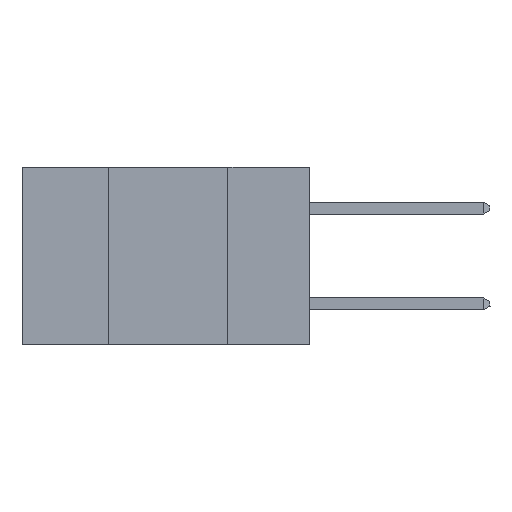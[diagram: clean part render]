
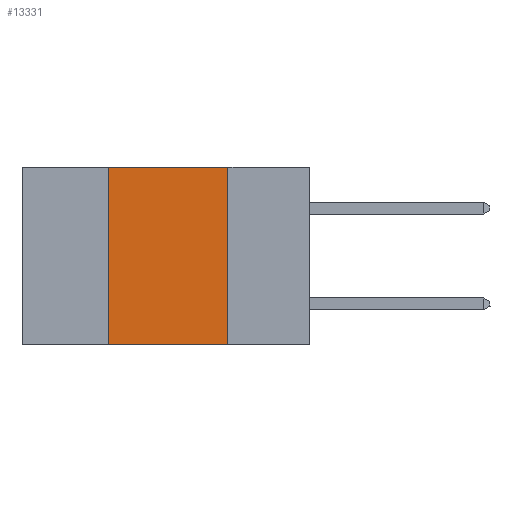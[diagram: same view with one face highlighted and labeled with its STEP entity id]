
A CAD part, left-side view. The second image highlights one B-rep face of the part: STEP entity #13331.
In plain terms, the highlighted planar face has unit normal (-1, 0, 0).
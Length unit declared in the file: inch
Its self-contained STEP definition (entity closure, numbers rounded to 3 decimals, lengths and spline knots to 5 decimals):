
#388 = ORIENTED_EDGE ( 'NONE', *, *, #21120, .T. ) ;
#2815 = VERTEX_POINT ( 'NONE', #7739 ) ;
#3692 = LINE ( 'NONE', #8326, #28881 ) ;
#4104 = CARTESIAN_POINT ( 'NONE',  ( 0., 0.42, -0.37 ) ) ;
#4304 = VERTEX_POINT ( 'NONE', #4104 ) ;
#4949 = ORIENTED_EDGE ( 'NONE', *, *, #5850, .F. ) ;
#5343 = CARTESIAN_POINT ( 'NONE',  ( 0., 0.6, 0. ) ) ;
#5487 = FACE_OUTER_BOUND ( 'NONE', #8391, .T. ) ;
#5850 = EDGE_CURVE ( 'NONE', #20703, #7345, #31725, .T. ) ;
#6881 = VECTOR ( 'NONE', #29168, 39.37008 ) ;
#7345 = VERTEX_POINT ( 'NONE', #27396 ) ;
#7739 = CARTESIAN_POINT ( 'NONE',  ( 0., 0.42, 0. ) ) ;
#8326 = CARTESIAN_POINT ( 'NONE',  ( 0., 0.6, -0.37 ) ) ;
#8391 = EDGE_LOOP ( 'NONE', ( #4949, #39964, #9537, #388 ) ) ;
#9324 = EDGE_CURVE ( 'NONE', #2815, #20703, #25489, .T. ) ;
#9537 = ORIENTED_EDGE ( 'NONE', *, *, #14345, .F. ) ;
#10808 = CARTESIAN_POINT ( 'NONE',  ( 0., 0.42, 0. ) ) ;
#10848 = LINE ( 'NONE', #10808, #6881 ) ;
#13331 = ADVANCED_FACE ( 'NONE', ( #5487 ), #30493, .F. ) ;
#14345 = EDGE_CURVE ( 'NONE', #4304, #2815, #10848, .T. ) ;
#15258 = DIRECTION ( 'NONE',  ( 1., 0., 0. ) ) ;
#17089 = VECTOR ( 'NONE', #21813, 39.37008 ) ;
#20703 = VERTEX_POINT ( 'NONE', #28363 ) ;
#21120 = EDGE_CURVE ( 'NONE', #4304, #7345, #3692, .T. ) ;
#21813 = DIRECTION ( 'NONE',  ( 0., -1., 0. ) ) ;
#25489 = LINE ( 'NONE', #34429, #17089 ) ;
#27319 = DIRECTION ( 'NONE',  ( 0., 0., -1. ) ) ;
#27396 = CARTESIAN_POINT ( 'NONE',  ( 0., 0.17, -0.37 ) ) ;
#28363 = CARTESIAN_POINT ( 'NONE',  ( 0., 0.17, 0. ) ) ;
#28881 = VECTOR ( 'NONE', #33186, 39.37008 ) ;
#29168 = DIRECTION ( 'NONE',  ( 0., 0., 1. ) ) ;
#30493 = PLANE ( 'NONE',  #37790 ) ;
#31725 = LINE ( 'NONE', #31810, #38660 ) ;
#31810 = CARTESIAN_POINT ( 'NONE',  ( 0., 0.17, 0. ) ) ;
#33186 = DIRECTION ( 'NONE',  ( 0., -1., 0. ) ) ;
#34429 = CARTESIAN_POINT ( 'NONE',  ( 0., 0.6, 0. ) ) ;
#34996 = DIRECTION ( 'NONE',  ( 0., 0., -1. ) ) ;
#37790 = AXIS2_PLACEMENT_3D ( 'NONE', #5343, #15258, #27319 ) ;
#38660 = VECTOR ( 'NONE', #34996, 39.37008 ) ;
#39964 = ORIENTED_EDGE ( 'NONE', *, *, #9324, .F. ) ;
